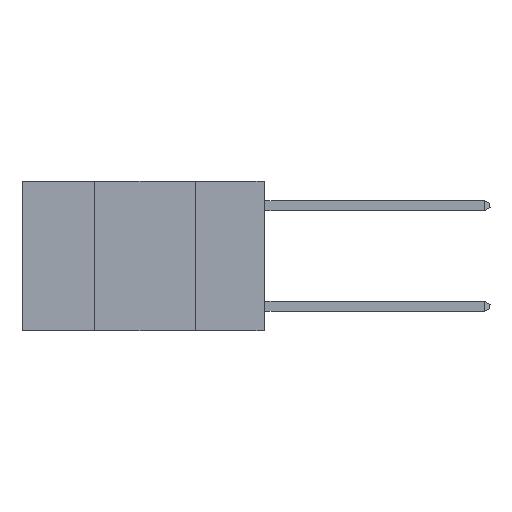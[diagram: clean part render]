
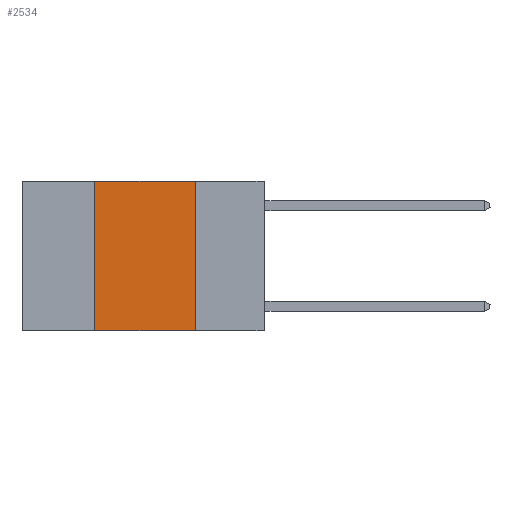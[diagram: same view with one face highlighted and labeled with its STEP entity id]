
A CAD part, left-side view. The second image highlights one B-rep face of the part: STEP entity #2534.
In plain terms, the highlighted planar face has unit normal (-1, 0, 0).
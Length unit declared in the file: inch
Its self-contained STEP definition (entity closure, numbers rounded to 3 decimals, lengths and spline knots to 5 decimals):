
#301 = CARTESIAN_POINT ( 'NONE',  ( 0., 0.17, 0. ) ) ;
#869 = CARTESIAN_POINT ( 'NONE',  ( 0., 0.6, -0.37 ) ) ;
#1654 = VECTOR ( 'NONE', #2996, 39.37008 ) ;
#2387 = EDGE_CURVE ( 'NONE', #6387, #10469, #6961, .T. ) ;
#2534 = ADVANCED_FACE ( 'NONE', ( #9602 ), #9231, .F. ) ;
#2996 = DIRECTION ( 'NONE',  ( 0., 0., -1. ) ) ;
#3692 = EDGE_CURVE ( 'NONE', #6387, #11541, #4848, .T. ) ;
#3991 = LINE ( 'NONE', #12014, #1654 ) ;
#4288 = DIRECTION ( 'NONE',  ( 0., -1., 0. ) ) ;
#4352 = EDGE_CURVE ( 'NONE', #10469, #4782, #5222, .T. ) ;
#4517 = CARTESIAN_POINT ( 'NONE',  ( 0., 0.42, -0.37 ) ) ;
#4538 = ORIENTED_EDGE ( 'NONE', *, *, #2387, .F. ) ;
#4782 = VERTEX_POINT ( 'NONE', #301 ) ;
#4848 = LINE ( 'NONE', #869, #10502 ) ;
#5222 = LINE ( 'NONE', #9287, #6490 ) ;
#5553 = ORIENTED_EDGE ( 'NONE', *, *, #3692, .T. ) ;
#6387 = VERTEX_POINT ( 'NONE', #4517 ) ;
#6490 = VECTOR ( 'NONE', #4288, 39.37008 ) ;
#6961 = LINE ( 'NONE', #10104, #11660 ) ;
#7292 = EDGE_LOOP ( 'NONE', ( #11579, #10596, #4538, #5553 ) ) ;
#9231 = PLANE ( 'NONE',  #9780 ) ;
#9287 = CARTESIAN_POINT ( 'NONE',  ( 0., 0.6, 0. ) ) ;
#9528 = DIRECTION ( 'NONE',  ( 0., 0., -1. ) ) ;
#9602 = FACE_OUTER_BOUND ( 'NONE', #7292, .T. ) ;
#9669 = DIRECTION ( 'NONE',  ( 1., 0., 0. ) ) ;
#9780 = AXIS2_PLACEMENT_3D ( 'NONE', #12312, #9669, #9528 ) ;
#9906 = DIRECTION ( 'NONE',  ( 0., 0., 1. ) ) ;
#10104 = CARTESIAN_POINT ( 'NONE',  ( 0., 0.42, 0. ) ) ;
#10469 = VERTEX_POINT ( 'NONE', #11875 ) ;
#10502 = VECTOR ( 'NONE', #11670, 39.37008 ) ;
#10596 = ORIENTED_EDGE ( 'NONE', *, *, #4352, .F. ) ;
#11116 = CARTESIAN_POINT ( 'NONE',  ( 0., 0.17, -0.37 ) ) ;
#11464 = EDGE_CURVE ( 'NONE', #4782, #11541, #3991, .T. ) ;
#11541 = VERTEX_POINT ( 'NONE', #11116 ) ;
#11579 = ORIENTED_EDGE ( 'NONE', *, *, #11464, .F. ) ;
#11660 = VECTOR ( 'NONE', #9906, 39.37008 ) ;
#11670 = DIRECTION ( 'NONE',  ( 0., -1., 0. ) ) ;
#11875 = CARTESIAN_POINT ( 'NONE',  ( 0., 0.42, 0. ) ) ;
#12014 = CARTESIAN_POINT ( 'NONE',  ( 0., 0.17, 0. ) ) ;
#12312 = CARTESIAN_POINT ( 'NONE',  ( 0., 0.6, 0. ) ) ;
